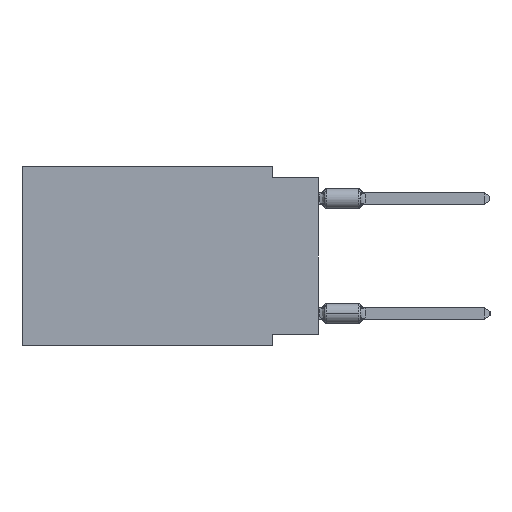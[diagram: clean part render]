
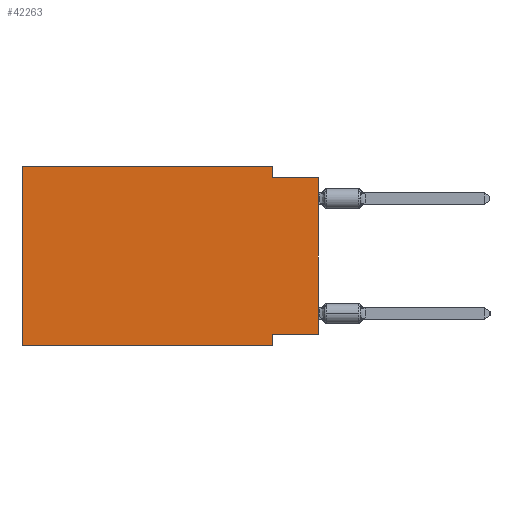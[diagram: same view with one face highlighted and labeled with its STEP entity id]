
A CAD part, left-side view. The second image highlights one B-rep face of the part: STEP entity #42263.
In plain terms, the highlighted planar face has unit normal (-1, 0, 0).
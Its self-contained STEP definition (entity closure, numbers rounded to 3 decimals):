
#734 = VERTEX_POINT ( 'NONE', #35595 ) ;
#987 = DIRECTION ( 'NONE',  ( 0., 1., 0. ) ) ;
#1607 = EDGE_CURVE ( 'NONE', #37788, #15830, #24485, .T. ) ;
#2479 = CARTESIAN_POINT ( 'NONE',  ( 0., 16.383, 0. ) ) ;
#2939 = EDGE_CURVE ( 'NONE', #8130, #39099, #37477, .T. ) ;
#3026 = EDGE_CURVE ( 'NONE', #8130, #8026, #24936, .T. ) ;
#4200 = LINE ( 'NONE', #18598, #10787 ) ;
#5928 = LINE ( 'NONE', #2479, #21068 ) ;
#6784 = VECTOR ( 'NONE', #31254, 1000. ) ;
#7010 = LINE ( 'NONE', #38554, #6784 ) ;
#7132 = DIRECTION ( 'NONE',  ( 0., 0., -1. ) ) ;
#8026 = VERTEX_POINT ( 'NONE', #36492 ) ;
#8130 = VERTEX_POINT ( 'NONE', #12031 ) ;
#9370 = DIRECTION ( 'NONE',  ( 0., -1., 0. ) ) ;
#9645 = CARTESIAN_POINT ( 'NONE',  ( 0., 16.383, 0. ) ) ;
#9681 = EDGE_CURVE ( 'NONE', #36662, #8026, #29575, .T. ) ;
#9999 = ORIENTED_EDGE ( 'NONE', *, *, #21227, .F. ) ;
#10266 = CARTESIAN_POINT ( 'NONE',  ( 0., 16.383, -9.906 ) ) ;
#10787 = VECTOR ( 'NONE', #987, 1000. ) ;
#12031 = CARTESIAN_POINT ( 'NONE',  ( 0., 16.383, -9.906 ) ) ;
#12087 = VECTOR ( 'NONE', #34274, 1000. ) ;
#12445 = CARTESIAN_POINT ( 'NONE',  ( 0., 2.54, -9.271 ) ) ;
#14735 = CARTESIAN_POINT ( 'NONE',  ( 0., 2.54, -9.906 ) ) ;
#15830 = VERTEX_POINT ( 'NONE', #42787 ) ;
#16391 = LINE ( 'NONE', #27795, #31847 ) ;
#17587 = ORIENTED_EDGE ( 'NONE', *, *, #23027, .F. ) ;
#18472 = VECTOR ( 'NONE', #36442, 1000. ) ;
#18598 = CARTESIAN_POINT ( 'NONE',  ( 0., 0., -9.271 ) ) ;
#21068 = VECTOR ( 'NONE', #9370, 1000. ) ;
#21227 = EDGE_CURVE ( 'NONE', #15830, #734, #16391, .T. ) ;
#23027 = EDGE_CURVE ( 'NONE', #32628, #36662, #4200, .T. ) ;
#24208 = DIRECTION ( 'NONE',  ( 0., -1., 0. ) ) ;
#24485 = LINE ( 'NONE', #24720, #30993 ) ;
#24720 = CARTESIAN_POINT ( 'NONE',  ( 0., 2.54, 0. ) ) ;
#24936 = LINE ( 'NONE', #10266, #35452 ) ;
#25763 = EDGE_CURVE ( 'NONE', #32628, #734, #7010, .T. ) ;
#25932 = ORIENTED_EDGE ( 'NONE', *, *, #2939, .F. ) ;
#27767 = ORIENTED_EDGE ( 'NONE', *, *, #25763, .T. ) ;
#27795 = CARTESIAN_POINT ( 'NONE',  ( 0., 0., -0.635 ) ) ;
#28817 = CARTESIAN_POINT ( 'NONE',  ( 0., 0., -9.271 ) ) ;
#29006 = CARTESIAN_POINT ( 'NONE',  ( 0., 2.54, 0. ) ) ;
#29575 = LINE ( 'NONE', #14735, #18472 ) ;
#29827 = ORIENTED_EDGE ( 'NONE', *, *, #40748, .F. ) ;
#30849 = CARTESIAN_POINT ( 'NONE',  ( 0., 16.383, 0. ) ) ;
#30993 = VECTOR ( 'NONE', #38662, 1000. ) ;
#31254 = DIRECTION ( 'NONE',  ( 0., 0., 1. ) ) ;
#31847 = VECTOR ( 'NONE', #45172, 1000. ) ;
#32628 = VERTEX_POINT ( 'NONE', #28817 ) ;
#34274 = DIRECTION ( 'NONE',  ( 0., 0., 1. ) ) ;
#34807 = ORIENTED_EDGE ( 'NONE', *, *, #9681, .F. ) ;
#35452 = VECTOR ( 'NONE', #24208, 1000. ) ;
#35595 = CARTESIAN_POINT ( 'NONE',  ( 0., 0., -0.635 ) ) ;
#36442 = DIRECTION ( 'NONE',  ( 0., 0., -1. ) ) ;
#36492 = CARTESIAN_POINT ( 'NONE',  ( 0., 2.54, -9.906 ) ) ;
#36662 = VERTEX_POINT ( 'NONE', #12445 ) ;
#37277 = EDGE_LOOP ( 'NONE', ( #27767, #9999, #37938, #29827, #25932, #41840, #34807, #17587 ) ) ;
#37477 = LINE ( 'NONE', #30849, #12087 ) ;
#37533 = DIRECTION ( 'NONE',  ( 1., 0., 0. ) ) ;
#37788 = VERTEX_POINT ( 'NONE', #29006 ) ;
#37938 = ORIENTED_EDGE ( 'NONE', *, *, #1607, .F. ) ;
#38554 = CARTESIAN_POINT ( 'NONE',  ( 0., 0., 0. ) ) ;
#38662 = DIRECTION ( 'NONE',  ( 0., 0., -1. ) ) ;
#39099 = VERTEX_POINT ( 'NONE', #39525 ) ;
#39525 = CARTESIAN_POINT ( 'NONE',  ( 0., 16.383, 0. ) ) ;
#40748 = EDGE_CURVE ( 'NONE', #39099, #37788, #5928, .T. ) ;
#40983 = PLANE ( 'NONE',  #45149 ) ;
#41840 = ORIENTED_EDGE ( 'NONE', *, *, #3026, .T. ) ;
#42263 = ADVANCED_FACE ( 'NONE', ( #44405 ), #40983, .F. ) ;
#42787 = CARTESIAN_POINT ( 'NONE',  ( 0., 2.54, -0.635 ) ) ;
#44405 = FACE_OUTER_BOUND ( 'NONE', #37277, .T. ) ;
#45149 = AXIS2_PLACEMENT_3D ( 'NONE', #9645, #37533, #7132 ) ;
#45172 = DIRECTION ( 'NONE',  ( 0., -1., 0. ) ) ;
